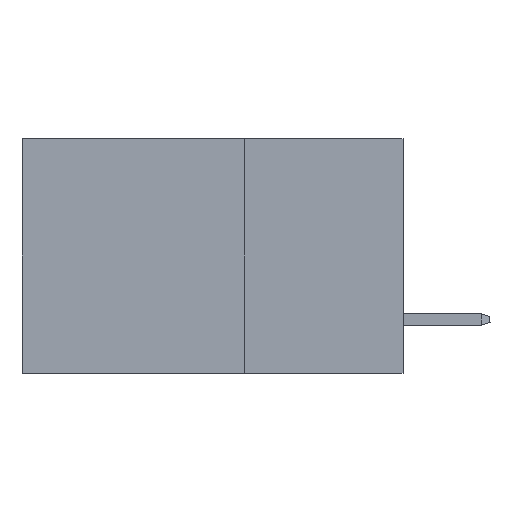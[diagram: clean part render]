
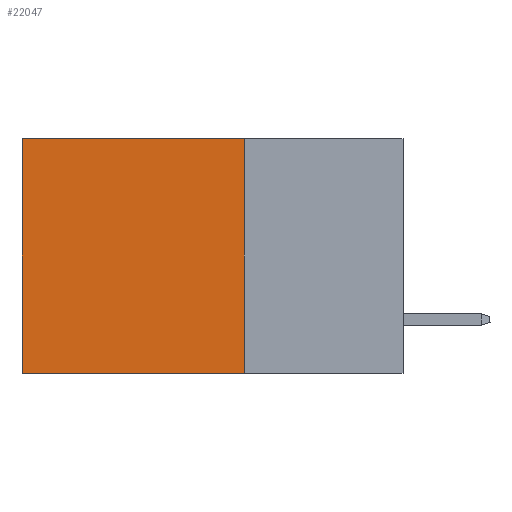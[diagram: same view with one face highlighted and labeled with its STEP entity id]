
A CAD part, left-side view. The second image highlights one B-rep face of the part: STEP entity #22047.
In plain terms, the highlighted planar face has unit normal (-1, 0, 0).
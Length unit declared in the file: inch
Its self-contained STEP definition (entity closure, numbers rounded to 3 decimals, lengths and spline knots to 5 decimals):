
#126 = EDGE_CURVE ( 'NONE', #9514, #30558, #3490, .T. ) ;
#1311 = EDGE_CURVE ( 'NONE', #2862, #15892, #10197, .T. ) ;
#1658 = CARTESIAN_POINT ( 'NONE',  ( 0.2875, 0.6, 0. ) ) ;
#2862 = VERTEX_POINT ( 'NONE', #22111 ) ;
#3063 = CARTESIAN_POINT ( 'NONE',  ( 0.2875, 0.25, -0.37 ) ) ;
#3382 = EDGE_LOOP ( 'NONE', ( #5448, #9813, #12979, #17250 ) ) ;
#3490 = LINE ( 'NONE', #8950, #12232 ) ;
#3761 = EDGE_CURVE ( 'NONE', #15892, #30558, #29598, .T. ) ;
#4425 = VECTOR ( 'NONE', #16458, 39.37008 ) ;
#5377 = VECTOR ( 'NONE', #7030, 39.37008 ) ;
#5448 = ORIENTED_EDGE ( 'NONE', *, *, #126, .T. ) ;
#5726 = CARTESIAN_POINT ( 'NONE',  ( 0.2875, 0.25, 0. ) ) ;
#7030 = DIRECTION ( 'NONE',  ( 0., 0., -1. ) ) ;
#8942 = AXIS2_PLACEMENT_3D ( 'NONE', #33306, #24715, #28068 ) ;
#8950 = CARTESIAN_POINT ( 'NONE',  ( 0.2875, 0.6, 0. ) ) ;
#9250 = EDGE_CURVE ( 'NONE', #2862, #9514, #32284, .T. ) ;
#9514 = VERTEX_POINT ( 'NONE', #1658 ) ;
#9813 = ORIENTED_EDGE ( 'NONE', *, *, #3761, .F. ) ;
#10197 = LINE ( 'NONE', #23057, #5377 ) ;
#12232 = VECTOR ( 'NONE', #17389, 39.37008 ) ;
#12979 = ORIENTED_EDGE ( 'NONE', *, *, #1311, .F. ) ;
#14473 = FACE_OUTER_BOUND ( 'NONE', #3382, .T. ) ;
#15892 = VERTEX_POINT ( 'NONE', #3063 ) ;
#16458 = DIRECTION ( 'NONE',  ( 0., 1., 0. ) ) ;
#17250 = ORIENTED_EDGE ( 'NONE', *, *, #9250, .T. ) ;
#17389 = DIRECTION ( 'NONE',  ( 0., 0., -1. ) ) ;
#18142 = CARTESIAN_POINT ( 'NONE',  ( 0.2875, 0.6, -0.37 ) ) ;
#20973 = DIRECTION ( 'NONE',  ( 0., 1., 0. ) ) ;
#22047 = ADVANCED_FACE ( 'NONE', ( #14473 ), #32962, .F. ) ;
#22111 = CARTESIAN_POINT ( 'NONE',  ( 0.2875, 0.25, 0. ) ) ;
#23057 = CARTESIAN_POINT ( 'NONE',  ( 0.2875, 0.25, 0. ) ) ;
#24715 = DIRECTION ( 'NONE',  ( 1., 0., 0. ) ) ;
#26263 = CARTESIAN_POINT ( 'NONE',  ( 0.2875, 0.25, -0.37 ) ) ;
#27144 = VECTOR ( 'NONE', #20973, 39.37008 ) ;
#28068 = DIRECTION ( 'NONE',  ( 0., 0., -1. ) ) ;
#29598 = LINE ( 'NONE', #26263, #27144 ) ;
#30558 = VERTEX_POINT ( 'NONE', #18142 ) ;
#32284 = LINE ( 'NONE', #5726, #4425 ) ;
#32962 = PLANE ( 'NONE',  #8942 ) ;
#33306 = CARTESIAN_POINT ( 'NONE',  ( 0.2875, 0.25, 0. ) ) ;
